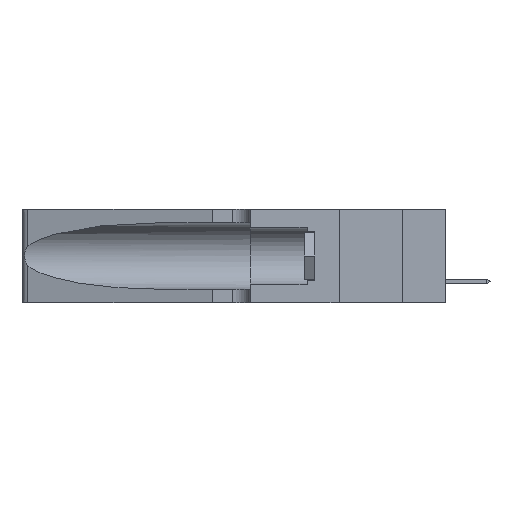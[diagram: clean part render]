
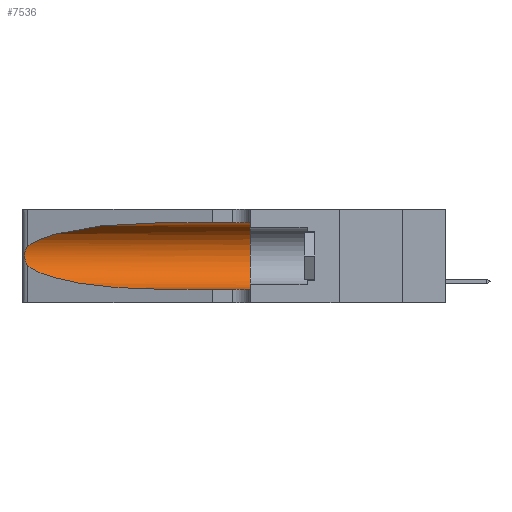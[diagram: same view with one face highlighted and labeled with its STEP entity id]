
A CAD part, left-side view. The second image highlights one B-rep face of the part: STEP entity #7536.
In plain terms, the highlighted cylindrical face has radius 3.308 mm (diameter 6.617 mm), a partial arc.
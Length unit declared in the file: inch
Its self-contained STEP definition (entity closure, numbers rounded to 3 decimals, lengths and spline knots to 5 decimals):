
#86 = CARTESIAN_POINT ( 'NONE',  ( 0.25856, 1.23593, 0.16098 ) ) ;
#223 = EDGE_CURVE ( 'NONE', #5201, #27835, #26319, .T. ) ;
#241 = ORIENTED_EDGE ( 'NONE', *, *, #223, .T. ) ;
#368 = FACE_OUTER_BOUND ( 'NONE', #8875, .T. ) ;
#5201 = VERTEX_POINT ( 'NONE', #26030 ) ;
#5337 = VECTOR ( 'NONE', #16082, 39.37008 ) ;
#5412 = CARTESIAN_POINT ( 'NONE',  ( 0.25789, 1.23486, 0.15765 ) ) ;
#5889 = EDGE_CURVE ( 'NONE', #17868, #26761, #21858, .T. ) ;
#6326 = CARTESIAN_POINT ( 'NONE',  ( 0.1305, 0.35, 0.185 ) ) ;
#6733 = AXIS2_PLACEMENT_3D ( 'NONE', #6326, #30482, #8779 ) ;
#6998 = CARTESIAN_POINT ( 'NONE',  ( 0.1305, 0.72297, 0.31525 ) ) ;
#7206 = CARTESIAN_POINT ( 'NONE',  ( 0.25487, 1.22718, 0.14631 ) ) ;
#7379 = ORIENTED_EDGE ( 'NONE', *, *, #31412, .T. ) ;
#7536 = ADVANCED_FACE ( 'NONE', ( #368 ), #16040, .F. ) ;
#7659 = CARTESIAN_POINT ( 'NONE',  ( 0.25639, 1.23186, 0.15144 ) ) ;
#7683 = CARTESIAN_POINT ( 'NONE',  ( 0.18966, 0.96281, 0.31525 ) ) ;
#7866 = CARTESIAN_POINT ( 'NONE',  ( 0.25487, 1.22718, 0.22369 ) ) ;
#8617 = EDGE_CURVE ( 'NONE', #17868, #18918, #20520, .T. ) ;
#8779 = DIRECTION ( 'NONE',  ( 0., 0., 1. ) ) ;
#8875 = EDGE_LOOP ( 'NONE', ( #19626, #7379, #16596, #241, #9488, #16942 ) ) ;
#9488 = ORIENTED_EDGE ( 'NONE', *, *, #26182, .F. ) ;
#10004 = CARTESIAN_POINT ( 'NONE',  ( 0.26075, 1.23896, 0.19203 ) ) ;
#10216 = CARTESIAN_POINT ( 'NONE',  ( 0.25555, 1.22994, 0.2215 ) ) ;
#10315 = CARTESIAN_POINT ( 'NONE',  ( 0.25639, 1.23184, 0.21858 ) ) ;
#11579 = DIRECTION ( 'NONE',  ( 0., -1., 0. ) ) ;
#12214 = CARTESIAN_POINT ( 'NONE',  ( 0.1305, 0.72297, 0.05475 ) ) ;
#13292 = CIRCLE ( 'NONE', #6733, 0.13025 ) ;
#15981 = VERTEX_POINT ( 'NONE', #26732 ) ;
#16040 = CYLINDRICAL_SURFACE ( 'NONE', #17495, 0.13025 ) ;
#16082 = DIRECTION ( 'NONE',  ( 0., -1., 0. ) ) ;
#16596 = ORIENTED_EDGE ( 'NONE', *, *, #24640, .T. ) ;
#16942 = ORIENTED_EDGE ( 'NONE', *, *, #5889, .F. ) ;
#17016 = CARTESIAN_POINT ( 'NONE',  ( 0.2373, 1.15595, 0.08982 ) ) ;
#17489 = CARTESIAN_POINT ( 'NONE',  ( 0.1305, 0.72297, 0.31525 ) ) ;
#17495 = AXIS2_PLACEMENT_3D ( 'NONE', #26273, #11579, #28591 ) ;
#17868 = VERTEX_POINT ( 'NONE', #6998 ) ;
#18918 = VERTEX_POINT ( 'NONE', #23354 ) ;
#19626 = ORIENTED_EDGE ( 'NONE', *, *, #8617, .T. ) ;
#19703 = CARTESIAN_POINT ( 'NONE',  ( 0.25555, 1.22993, 0.14849 ) ) ;
#19729 = CARTESIAN_POINT ( 'NONE',  ( 0.25487, 1.22718, 0.22369 ) ) ;
#19909 = CARTESIAN_POINT ( 'NONE',  ( 0.26018, 1.23835, 0.19895 ) ) ;
#20084 = CARTESIAN_POINT ( 'NONE',  ( 0.1305, 1.61858, 0.31525 ) ) ;
#20520 =( BOUNDED_CURVE ( )  B_SPLINE_CURVE ( 3, ( #17489, #7683, #29597, #19729 ),
 .UNSPECIFIED., .F., .F. ) 
 B_SPLINE_CURVE_WITH_KNOTS ( ( 4, 4 ),
 ( 1.5708, 2.84003 ),
 .UNSPECIFIED. ) 
 CURVE ( )  GEOMETRIC_REPRESENTATION_ITEM ( )  RATIONAL_B_SPLINE_CURVE ( ( 1., 0.87, 0.87, 1. ) ) 
 REPRESENTATION_ITEM ( '' )  );
#21290 = CARTESIAN_POINT ( 'NONE',  ( 0.1305, 1.61858, 0.05475 ) ) ;
#21515 =( BOUNDED_CURVE ( )  B_SPLINE_CURVE ( 3, ( #7206, #17016, #24054, #12214 ),
 .UNSPECIFIED., .F., .F. ) 
 B_SPLINE_CURVE_WITH_KNOTS ( ( 4, 4 ),
 ( 3.44316, 4.71239 ),
 .UNSPECIFIED. ) 
 CURVE ( )  GEOMETRIC_REPRESENTATION_ITEM ( )  RATIONAL_B_SPLINE_CURVE ( ( 1., 0.87, 0.87, 1. ) ) 
 REPRESENTATION_ITEM ( '' )  );
#21858 = LINE ( 'NONE', #20084, #22986 ) ;
#22040 = CARTESIAN_POINT ( 'NONE',  ( 0.25854, 1.2359, 0.20912 ) ) ;
#22986 = VECTOR ( 'NONE', #27661, 39.37008 ) ;
#23354 = CARTESIAN_POINT ( 'NONE',  ( 0.25487, 1.22718, 0.22369 ) ) ;
#24054 = CARTESIAN_POINT ( 'NONE',  ( 0.18966, 0.96281, 0.05475 ) ) ;
#24640 = EDGE_CURVE ( 'NONE', #15981, #5201, #21515, .T. ) ;
#24898 = CARTESIAN_POINT ( 'NONE',  ( 0.26017, 1.23833, 0.17102 ) ) ;
#26030 = CARTESIAN_POINT ( 'NONE',  ( 0.1305, 0.72297, 0.05475 ) ) ;
#26182 = EDGE_CURVE ( 'NONE', #26761, #27835, #13292, .T. ) ;
#26273 = CARTESIAN_POINT ( 'NONE',  ( 0.1305, 1.61858, 0.185 ) ) ;
#26319 = LINE ( 'NONE', #21290, #5337 ) ;
#26732 = CARTESIAN_POINT ( 'NONE',  ( 0.25487, 1.22718, 0.14631 ) ) ;
#26761 = VERTEX_POINT ( 'NONE', #30082 ) ;
#26783 = B_SPLINE_CURVE_WITH_KNOTS ( 'NONE', 3,
 ( #7866, #10216, #10315, #27265, #22040, #19909, #10004, #27162, #24898, #86, #5412, #7659, #19703, #27371 ),
 .UNSPECIFIED., .F., .F.,
 ( 4, 2, 2, 2, 2, 2, 4 ),
 ( 0., 0.00027, 0.00053, 0.00107, 0.0016, 0.00187, 0.00214 ),
 .UNSPECIFIED. ) ;
#27162 = CARTESIAN_POINT ( 'NONE',  ( 0.26075, 1.23896, 0.178 ) ) ;
#27182 = CARTESIAN_POINT ( 'NONE',  ( 0.1305, 0.35, 0.05475 ) ) ;
#27265 = CARTESIAN_POINT ( 'NONE',  ( 0.25787, 1.23484, 0.2124 ) ) ;
#27371 = CARTESIAN_POINT ( 'NONE',  ( 0.25487, 1.22718, 0.14631 ) ) ;
#27661 = DIRECTION ( 'NONE',  ( 0., -1., 0. ) ) ;
#27835 = VERTEX_POINT ( 'NONE', #27182 ) ;
#28591 = DIRECTION ( 'NONE',  ( 0., 0., -1. ) ) ;
#29597 = CARTESIAN_POINT ( 'NONE',  ( 0.2373, 1.15595, 0.28018 ) ) ;
#30082 = CARTESIAN_POINT ( 'NONE',  ( 0.1305, 0.35, 0.31525 ) ) ;
#30482 = DIRECTION ( 'NONE',  ( 0., 1., 0. ) ) ;
#31412 = EDGE_CURVE ( 'NONE', #18918, #15981, #26783, .T. ) ;
